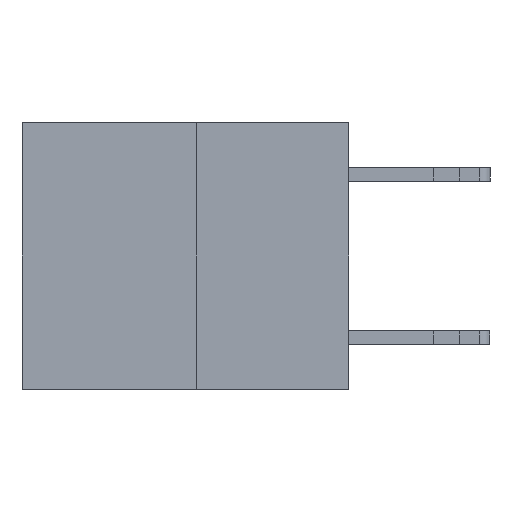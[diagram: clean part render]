
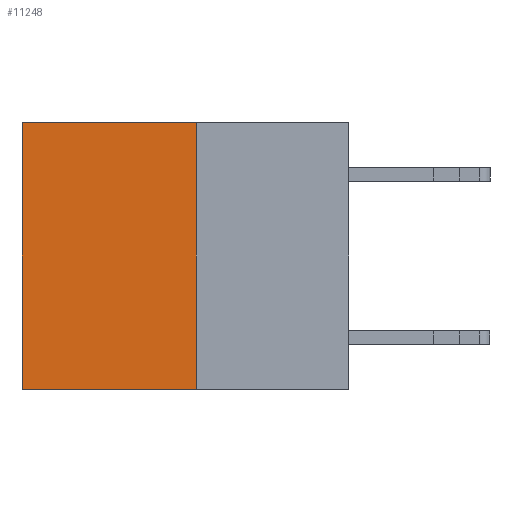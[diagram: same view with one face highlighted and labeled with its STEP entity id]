
A CAD part, left-side view. The second image highlights one B-rep face of the part: STEP entity #11248.
In plain terms, the highlighted planar face has unit normal (-1, 0, 0).
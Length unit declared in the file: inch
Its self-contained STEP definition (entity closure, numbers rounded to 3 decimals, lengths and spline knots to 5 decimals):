
#244 = CARTESIAN_POINT ( 'NONE',  ( 0.3165, 0.6, -0.49 ) ) ;
#315 = AXIS2_PLACEMENT_3D ( 'NONE', #4241, #7631, #971 ) ;
#617 = CARTESIAN_POINT ( 'NONE',  ( 0.3165, 0.28, -0.49 ) ) ;
#968 = VERTEX_POINT ( 'NONE', #617 ) ;
#971 = DIRECTION ( 'NONE',  ( 0., 0., -1. ) ) ;
#1563 = FACE_OUTER_BOUND ( 'NONE', #11089, .T. ) ;
#1808 = EDGE_CURVE ( 'NONE', #968, #13798, #2392, .T. ) ;
#2113 = EDGE_CURVE ( 'NONE', #11770, #13798, #3115, .T. ) ;
#2392 = LINE ( 'NONE', #12940, #14071 ) ;
#2599 = VERTEX_POINT ( 'NONE', #10833 ) ;
#2910 = ORIENTED_EDGE ( 'NONE', *, *, #10311, .T. ) ;
#3036 = DIRECTION ( 'NONE',  ( 0., 1., 0. ) ) ;
#3115 = LINE ( 'NONE', #12344, #14052 ) ;
#3188 = VECTOR ( 'NONE', #9011, 39.37008 ) ;
#3202 = ORIENTED_EDGE ( 'NONE', *, *, #2113, .T. ) ;
#3953 = CARTESIAN_POINT ( 'NONE',  ( 0.3165, 0.28, -0.49 ) ) ;
#4241 = CARTESIAN_POINT ( 'NONE',  ( 0.3165, 0.28, -0.49 ) ) ;
#4549 = DIRECTION ( 'NONE',  ( 0., 0., -1. ) ) ;
#5778 = ORIENTED_EDGE ( 'NONE', *, *, #1808, .F. ) ;
#6470 = ORIENTED_EDGE ( 'NONE', *, *, #11503, .F. ) ;
#6517 = PLANE ( 'NONE',  #315 ) ;
#7326 = VECTOR ( 'NONE', #11937, 39.37008 ) ;
#7631 = DIRECTION ( 'NONE',  ( 1., 0., 0. ) ) ;
#9011 = DIRECTION ( 'NONE',  ( 0., 1., 0. ) ) ;
#9674 = LINE ( 'NONE', #3953, #7326 ) ;
#10311 = EDGE_CURVE ( 'NONE', #2599, #11770, #13597, .T. ) ;
#10524 = CARTESIAN_POINT ( 'NONE',  ( 0.3165, 0.6, 0. ) ) ;
#10833 = CARTESIAN_POINT ( 'NONE',  ( 0.3165, 0.28, 0. ) ) ;
#11089 = EDGE_LOOP ( 'NONE', ( #3202, #5778, #6470, #2910 ) ) ;
#11248 = ADVANCED_FACE ( 'NONE', ( #1563 ), #6517, .F. ) ;
#11503 = EDGE_CURVE ( 'NONE', #2599, #968, #9674, .T. ) ;
#11770 = VERTEX_POINT ( 'NONE', #10524 ) ;
#11937 = DIRECTION ( 'NONE',  ( 0., 0., -1. ) ) ;
#12344 = CARTESIAN_POINT ( 'NONE',  ( 0.3165, 0.6, -0.49 ) ) ;
#12940 = CARTESIAN_POINT ( 'NONE',  ( 0.3165, 0.28, -0.49 ) ) ;
#13597 = LINE ( 'NONE', #14214, #3188 ) ;
#13798 = VERTEX_POINT ( 'NONE', #244 ) ;
#14052 = VECTOR ( 'NONE', #4549, 39.37008 ) ;
#14071 = VECTOR ( 'NONE', #3036, 39.37008 ) ;
#14214 = CARTESIAN_POINT ( 'NONE',  ( 0.3165, 0.28, 0. ) ) ;
